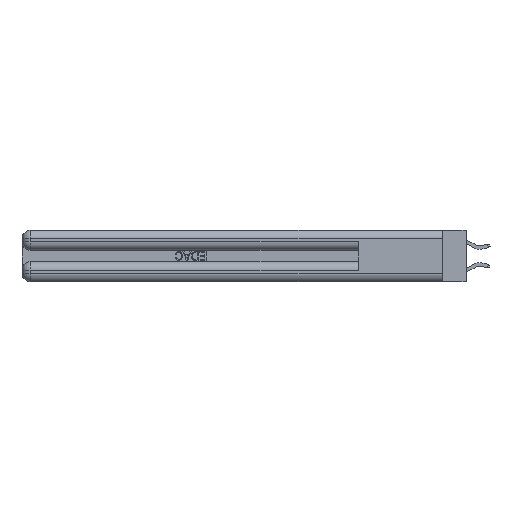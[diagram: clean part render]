
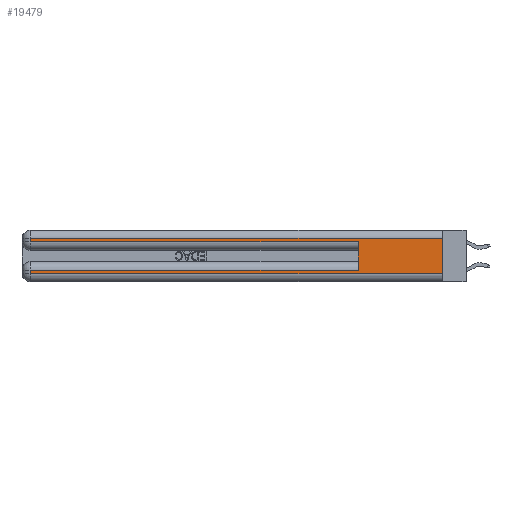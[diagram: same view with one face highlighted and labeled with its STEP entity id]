
A CAD part, left-side view. The second image highlights one B-rep face of the part: STEP entity #19479.
In plain terms, the highlighted planar face has unit normal (-1, 0, 0).
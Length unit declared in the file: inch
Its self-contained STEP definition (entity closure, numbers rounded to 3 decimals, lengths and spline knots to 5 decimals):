
#600 = CARTESIAN_POINT ( 'NONE',  ( 0., 2.94, 0.085 ) ) ;
#695 = CARTESIAN_POINT ( 'NONE',  ( 0., 2.94, 0.06 ) ) ;
#786 = VERTEX_POINT ( 'NONE', #30944 ) ;
#1402 = DIRECTION ( 'NONE',  ( 0., 1., 0. ) ) ;
#1910 = VECTOR ( 'NONE', #26866, 39.37008 ) ;
#2870 = DIRECTION ( 'NONE',  ( 0., 0., -1. ) ) ;
#3498 = VERTEX_POINT ( 'NONE', #695 ) ;
#4320 = CARTESIAN_POINT ( 'NONE',  ( 0., 0., 0.37 ) ) ;
#4525 = ORIENTED_EDGE ( 'NONE', *, *, #13080, .F. ) ;
#4742 = VECTOR ( 'NONE', #25289, 39.37008 ) ;
#4863 = ORIENTED_EDGE ( 'NONE', *, *, #16570, .T. ) ;
#6488 = CARTESIAN_POINT ( 'NONE',  ( 0., 2.94, 0.285 ) ) ;
#6593 = EDGE_CURVE ( 'NONE', #11252, #786, #31745, .T. ) ;
#6684 = ORIENTED_EDGE ( 'NONE', *, *, #33525, .T. ) ;
#8047 = ORIENTED_EDGE ( 'NONE', *, *, #6593, .F. ) ;
#8597 = CARTESIAN_POINT ( 'NONE',  ( 0., 0., 0.285 ) ) ;
#8896 = CARTESIAN_POINT ( 'NONE',  ( 0., 0., 0.31 ) ) ;
#9221 = VERTEX_POINT ( 'NONE', #25099 ) ;
#9669 = CARTESIAN_POINT ( 'NONE',  ( 0., 0., 0.31 ) ) ;
#9978 = VERTEX_POINT ( 'NONE', #17076 ) ;
#10087 = EDGE_CURVE ( 'NONE', #9978, #14964, #26768, .T. ) ;
#10162 = PLANE ( 'NONE',  #20509 ) ;
#10723 = LINE ( 'NONE', #9669, #32078 ) ;
#11214 = VECTOR ( 'NONE', #33135, 39.37008 ) ;
#11236 = FACE_OUTER_BOUND ( 'NONE', #28924, .T. ) ;
#11252 = VERTEX_POINT ( 'NONE', #8896 ) ;
#11893 = DIRECTION ( 'NONE',  ( 0., 1., 0. ) ) ;
#12704 = DIRECTION ( 'NONE',  ( 0., 0., -1. ) ) ;
#12966 = DIRECTION ( 'NONE',  ( 1., 0., 0. ) ) ;
#13080 = EDGE_CURVE ( 'NONE', #9978, #25837, #28410, .T. ) ;
#13569 = VECTOR ( 'NONE', #15015, 39.37008 ) ;
#13908 = VECTOR ( 'NONE', #2870, 39.37008 ) ;
#14964 = VERTEX_POINT ( 'NONE', #600 ) ;
#15015 = DIRECTION ( 'NONE',  ( 0., 0., 1. ) ) ;
#16570 = EDGE_CURVE ( 'NONE', #3498, #786, #33436, .T. ) ;
#17076 = CARTESIAN_POINT ( 'NONE',  ( 0., 0.6, 0.085 ) ) ;
#19372 = VECTOR ( 'NONE', #11893, 39.37008 ) ;
#19479 = ADVANCED_FACE ( 'NONE', ( #11236 ), #10162, .F. ) ;
#19598 = CARTESIAN_POINT ( 'NONE',  ( 0., 2.94, 0.37 ) ) ;
#20221 = CARTESIAN_POINT ( 'NONE',  ( 0., 0., 0.085 ) ) ;
#20509 = AXIS2_PLACEMENT_3D ( 'NONE', #29670, #12966, #32447 ) ;
#20633 = CARTESIAN_POINT ( 'NONE',  ( 0., 0.6, 0.145 ) ) ;
#21065 = ORIENTED_EDGE ( 'NONE', *, *, #28164, .T. ) ;
#24060 = CARTESIAN_POINT ( 'NONE',  ( 0., 2.94, 0.37 ) ) ;
#24140 = LINE ( 'NONE', #24060, #1910 ) ;
#25099 = CARTESIAN_POINT ( 'NONE',  ( 0., 2.94, 0.31 ) ) ;
#25205 = VECTOR ( 'NONE', #12704, 39.37008 ) ;
#25289 = DIRECTION ( 'NONE',  ( 0., -1., 0. ) ) ;
#25837 = VERTEX_POINT ( 'NONE', #33055 ) ;
#26768 = LINE ( 'NONE', #20221, #19372 ) ;
#26866 = DIRECTION ( 'NONE',  ( 0., 0., -1. ) ) ;
#27465 = ORIENTED_EDGE ( 'NONE', *, *, #33580, .T. ) ;
#28164 = EDGE_CURVE ( 'NONE', #14964, #3498, #24140, .T. ) ;
#28410 = LINE ( 'NONE', #20633, #13569 ) ;
#28672 = VERTEX_POINT ( 'NONE', #6488 ) ;
#28775 = ORIENTED_EDGE ( 'NONE', *, *, #10087, .T. ) ;
#28924 = EDGE_LOOP ( 'NONE', ( #8047, #33129, #6684, #27465, #4525, #28775, #21065, #4863 ) ) ;
#29670 = CARTESIAN_POINT ( 'NONE',  ( 0., 0., 0.37 ) ) ;
#30340 = CARTESIAN_POINT ( 'NONE',  ( 0., 0., 0.06 ) ) ;
#30944 = CARTESIAN_POINT ( 'NONE',  ( 0., 0., 0.06 ) ) ;
#31745 = LINE ( 'NONE', #4320, #25205 ) ;
#32078 = VECTOR ( 'NONE', #1402, 39.37008 ) ;
#32447 = DIRECTION ( 'NONE',  ( 0., 0., -1. ) ) ;
#33055 = CARTESIAN_POINT ( 'NONE',  ( 0., 0.6, 0.285 ) ) ;
#33129 = ORIENTED_EDGE ( 'NONE', *, *, #35342, .T. ) ;
#33135 = DIRECTION ( 'NONE',  ( 0., -1., 0. ) ) ;
#33436 = LINE ( 'NONE', #30340, #11214 ) ;
#33512 = LINE ( 'NONE', #8597, #4742 ) ;
#33525 = EDGE_CURVE ( 'NONE', #9221, #28672, #34393, .T. ) ;
#33580 = EDGE_CURVE ( 'NONE', #28672, #25837, #33512, .T. ) ;
#34393 = LINE ( 'NONE', #19598, #13908 ) ;
#35342 = EDGE_CURVE ( 'NONE', #11252, #9221, #10723, .T. ) ;
